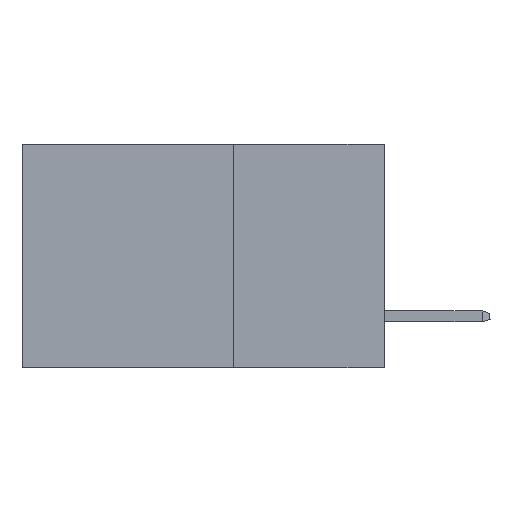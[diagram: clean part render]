
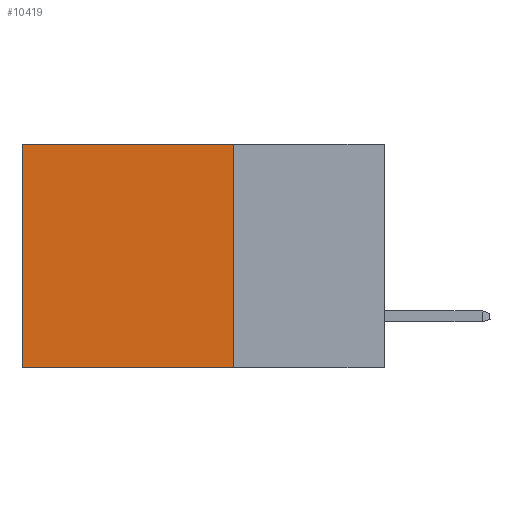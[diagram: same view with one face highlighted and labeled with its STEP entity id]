
A CAD part, left-side view. The second image highlights one B-rep face of the part: STEP entity #10419.
In plain terms, the highlighted planar face has unit normal (-1, 0, 0).
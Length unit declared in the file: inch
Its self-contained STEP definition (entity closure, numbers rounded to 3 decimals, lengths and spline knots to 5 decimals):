
#1208 = EDGE_CURVE ( 'NONE', #20823, #22493, #14448, .T. ) ;
#1512 = CARTESIAN_POINT ( 'NONE',  ( 0.298, 0.25, 0. ) ) ;
#2561 = VECTOR ( 'NONE', #11626, 39.37008 ) ;
#3764 = CARTESIAN_POINT ( 'NONE',  ( 0.298, 0.25, 0. ) ) ;
#4433 = DIRECTION ( 'NONE',  ( 0., 1., 0. ) ) ;
#4626 = ORIENTED_EDGE ( 'NONE', *, *, #29368, .F. ) ;
#7550 = VECTOR ( 'NONE', #18035, 39.37008 ) ;
#7580 = VERTEX_POINT ( 'NONE', #24938 ) ;
#10419 = ADVANCED_FACE ( 'NONE', ( #10544 ), #30079, .F. ) ;
#10544 = FACE_OUTER_BOUND ( 'NONE', #17887, .T. ) ;
#11626 = DIRECTION ( 'NONE',  ( 0., 0., -1. ) ) ;
#12803 = VECTOR ( 'NONE', #4433, 39.37008 ) ;
#13701 = VECTOR ( 'NONE', #29517, 39.37008 ) ;
#14448 = LINE ( 'NONE', #29732, #13701 ) ;
#14781 = LINE ( 'NONE', #21161, #2561 ) ;
#15379 = EDGE_CURVE ( 'NONE', #18465, #7580, #27667, .T. ) ;
#15709 = DIRECTION ( 'NONE',  ( 0., 0., -1. ) ) ;
#15757 = ORIENTED_EDGE ( 'NONE', *, *, #23118, .T. ) ;
#16033 = AXIS2_PLACEMENT_3D ( 'NONE', #1512, #27715, #15709 ) ;
#17887 = EDGE_LOOP ( 'NONE', ( #15757, #19017, #4626, #28263 ) ) ;
#18035 = DIRECTION ( 'NONE',  ( 0., 0., -1. ) ) ;
#18465 = VERTEX_POINT ( 'NONE', #27166 ) ;
#18556 = CARTESIAN_POINT ( 'NONE',  ( 0.298, 0.25, 0. ) ) ;
#19017 = ORIENTED_EDGE ( 'NONE', *, *, #15379, .F. ) ;
#20823 = VERTEX_POINT ( 'NONE', #18556 ) ;
#21161 = CARTESIAN_POINT ( 'NONE',  ( 0.298, 0.6, 0. ) ) ;
#21725 = CARTESIAN_POINT ( 'NONE',  ( 0.298, 0.6, 0. ) ) ;
#22493 = VERTEX_POINT ( 'NONE', #21725 ) ;
#23118 = EDGE_CURVE ( 'NONE', #22493, #7580, #14781, .T. ) ;
#23447 = CARTESIAN_POINT ( 'NONE',  ( 0.298, 0.25, -0.37 ) ) ;
#24938 = CARTESIAN_POINT ( 'NONE',  ( 0.298, 0.6, -0.37 ) ) ;
#24959 = LINE ( 'NONE', #3764, #7550 ) ;
#27166 = CARTESIAN_POINT ( 'NONE',  ( 0.298, 0.25, -0.37 ) ) ;
#27667 = LINE ( 'NONE', #23447, #12803 ) ;
#27715 = DIRECTION ( 'NONE',  ( 1., 0., 0. ) ) ;
#28263 = ORIENTED_EDGE ( 'NONE', *, *, #1208, .T. ) ;
#29368 = EDGE_CURVE ( 'NONE', #20823, #18465, #24959, .T. ) ;
#29517 = DIRECTION ( 'NONE',  ( 0., 1., 0. ) ) ;
#29732 = CARTESIAN_POINT ( 'NONE',  ( 0.298, 0.25, 0. ) ) ;
#30079 = PLANE ( 'NONE',  #16033 ) ;
